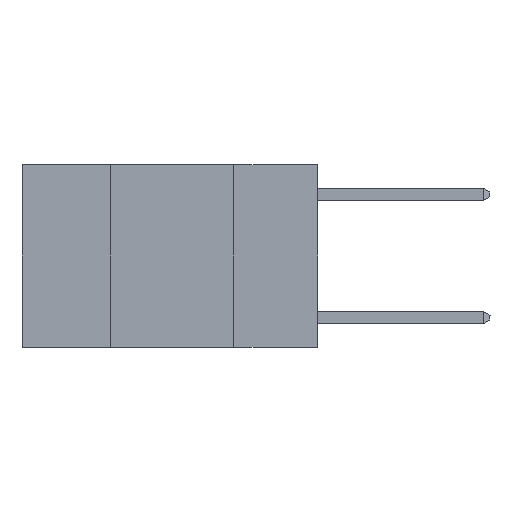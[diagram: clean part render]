
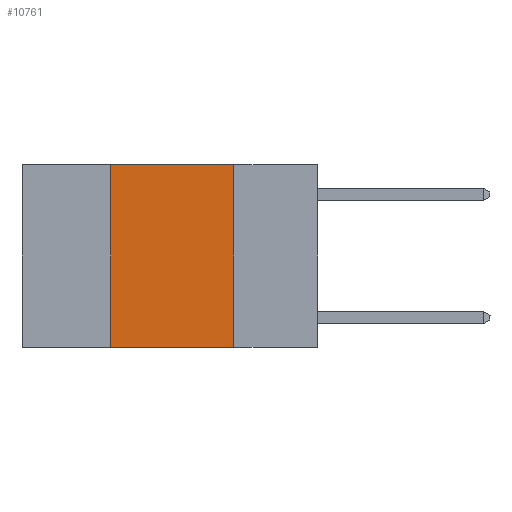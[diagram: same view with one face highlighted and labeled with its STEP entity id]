
A CAD part, left-side view. The second image highlights one B-rep face of the part: STEP entity #10761.
In plain terms, the highlighted planar face has unit normal (-1, 0, 0).
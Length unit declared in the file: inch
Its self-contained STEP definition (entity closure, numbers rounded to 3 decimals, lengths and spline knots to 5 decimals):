
#982 = PLANE ( 'NONE',  #3879 ) ;
#1585 = CARTESIAN_POINT ( 'NONE',  ( 0., 0.17, 0. ) ) ;
#1691 = EDGE_CURVE ( 'NONE', #7346, #2936, #10512, .T. ) ;
#1844 = EDGE_CURVE ( 'NONE', #4026, #11256, #9588, .T. ) ;
#2247 = ORIENTED_EDGE ( 'NONE', *, *, #3525, .F. ) ;
#2265 = CARTESIAN_POINT ( 'NONE',  ( 0., 0.17, -0.37 ) ) ;
#2280 = CARTESIAN_POINT ( 'NONE',  ( 0., 0.42, -0.37 ) ) ;
#2282 = ORIENTED_EDGE ( 'NONE', *, *, #1844, .F. ) ;
#2378 = ORIENTED_EDGE ( 'NONE', *, *, #2923, .F. ) ;
#2395 = ORIENTED_EDGE ( 'NONE', *, *, #1691, .T. ) ;
#2664 = DIRECTION ( 'NONE',  ( 0., -1., 0. ) ) ;
#2680 = CARTESIAN_POINT ( 'NONE',  ( 0., 0.6, 0. ) ) ;
#2844 = CARTESIAN_POINT ( 'NONE',  ( 0., 0.6, 0. ) ) ;
#2923 = EDGE_CURVE ( 'NONE', #7346, #4026, #10368, .T. ) ;
#2936 = VERTEX_POINT ( 'NONE', #2265 ) ;
#3137 = DIRECTION ( 'NONE',  ( 0., -1., 0. ) ) ;
#3228 = CARTESIAN_POINT ( 'NONE',  ( 0., 0.6, -0.37 ) ) ;
#3519 = VECTOR ( 'NONE', #3137, 39.37008 ) ;
#3525 = EDGE_CURVE ( 'NONE', #11256, #2936, #10651, .T. ) ;
#3752 = DIRECTION ( 'NONE',  ( 0., 0., -1. ) ) ;
#3879 = AXIS2_PLACEMENT_3D ( 'NONE', #2844, #9025, #3752 ) ;
#4026 = VERTEX_POINT ( 'NONE', #8508 ) ;
#4248 = EDGE_LOOP ( 'NONE', ( #2247, #2282, #2378, #2395 ) ) ;
#5750 = VECTOR ( 'NONE', #5848, 39.37008 ) ;
#5848 = DIRECTION ( 'NONE',  ( 0., 0., 1. ) ) ;
#6064 = VECTOR ( 'NONE', #11251, 39.37008 ) ;
#6207 = FACE_OUTER_BOUND ( 'NONE', #4248, .T. ) ;
#7346 = VERTEX_POINT ( 'NONE', #2280 ) ;
#8508 = CARTESIAN_POINT ( 'NONE',  ( 0., 0.42, 0. ) ) ;
#9025 = DIRECTION ( 'NONE',  ( 1., 0., 0. ) ) ;
#9326 = VECTOR ( 'NONE', #2664, 39.37008 ) ;
#9588 = LINE ( 'NONE', #2680, #9326 ) ;
#10368 = LINE ( 'NONE', #11025, #5750 ) ;
#10382 = CARTESIAN_POINT ( 'NONE',  ( 0., 0.17, 0. ) ) ;
#10512 = LINE ( 'NONE', #3228, #3519 ) ;
#10651 = LINE ( 'NONE', #10382, #6064 ) ;
#10761 = ADVANCED_FACE ( 'NONE', ( #6207 ), #982, .F. ) ;
#11025 = CARTESIAN_POINT ( 'NONE',  ( 0., 0.42, 0. ) ) ;
#11251 = DIRECTION ( 'NONE',  ( 0., 0., -1. ) ) ;
#11256 = VERTEX_POINT ( 'NONE', #1585 ) ;
